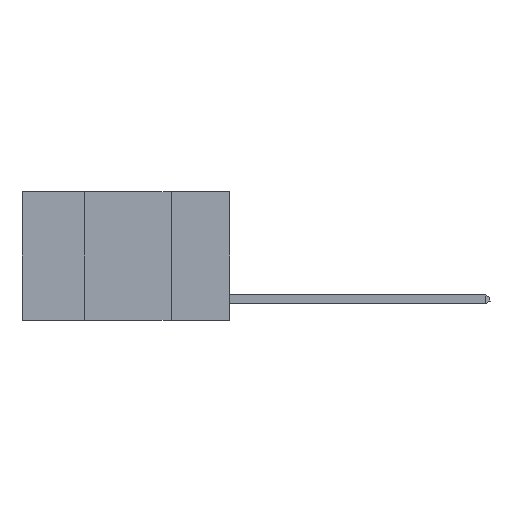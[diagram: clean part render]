
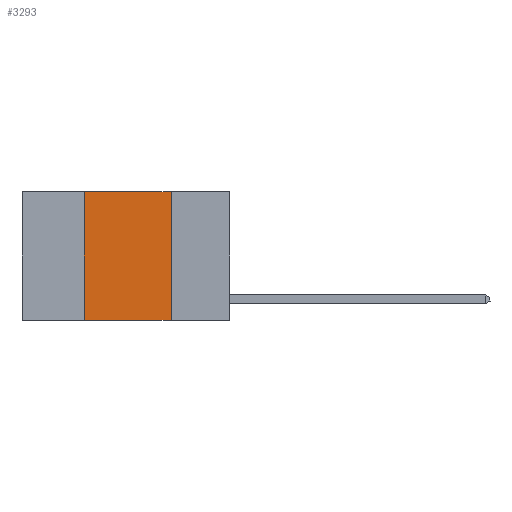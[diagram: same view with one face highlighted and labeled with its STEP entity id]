
A CAD part, left-side view. The second image highlights one B-rep face of the part: STEP entity #3293.
In plain terms, the highlighted planar face has unit normal (-1, 0, 0).
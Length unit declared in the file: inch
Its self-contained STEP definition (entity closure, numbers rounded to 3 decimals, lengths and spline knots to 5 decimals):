
#112 = AXIS2_PLACEMENT_3D ( 'NONE', #6970, #8048, #3590 ) ;
#480 = CARTESIAN_POINT ( 'NONE',  ( 0., 0.6, -0.37 ) ) ;
#869 = CARTESIAN_POINT ( 'NONE',  ( 0., 0.17, -0.37 ) ) ;
#885 = PLANE ( 'NONE',  #112 ) ;
#901 = ORIENTED_EDGE ( 'NONE', *, *, #1354, .F. ) ;
#1239 = LINE ( 'NONE', #4077, #8065 ) ;
#1354 = EDGE_CURVE ( 'NONE', #8734, #9245, #9266, .T. ) ;
#1361 = DIRECTION ( 'NONE',  ( 0., 0., -1. ) ) ;
#1508 = EDGE_CURVE ( 'NONE', #10641, #7084, #1239, .T. ) ;
#1574 = EDGE_LOOP ( 'NONE', ( #6700, #7855, #901, #9587 ) ) ;
#1585 = CARTESIAN_POINT ( 'NONE',  ( 0., 0.17, 0. ) ) ;
#2046 = VECTOR ( 'NONE', #9207, 39.37008 ) ;
#3048 = VECTOR ( 'NONE', #11203, 39.37008 ) ;
#3293 = ADVANCED_FACE ( 'NONE', ( #11440 ), #885, .F. ) ;
#3470 = VECTOR ( 'NONE', #4023, 39.37008 ) ;
#3590 = DIRECTION ( 'NONE',  ( 0., 0., -1. ) ) ;
#3980 = CARTESIAN_POINT ( 'NONE',  ( 0., 0.42, 0. ) ) ;
#4023 = DIRECTION ( 'NONE',  ( 0., -1., 0. ) ) ;
#4077 = CARTESIAN_POINT ( 'NONE',  ( 0., 0.17, 0. ) ) ;
#4091 = CARTESIAN_POINT ( 'NONE',  ( 0., 0.42, -0.37 ) ) ;
#4759 = CARTESIAN_POINT ( 'NONE',  ( 0., 0.6, 0. ) ) ;
#4962 = LINE ( 'NONE', #480, #3048 ) ;
#5036 = CARTESIAN_POINT ( 'NONE',  ( 0., 0.42, 0. ) ) ;
#6116 = EDGE_CURVE ( 'NONE', #8734, #7084, #4962, .T. ) ;
#6479 = LINE ( 'NONE', #4759, #3470 ) ;
#6700 = ORIENTED_EDGE ( 'NONE', *, *, #1508, .F. ) ;
#6970 = CARTESIAN_POINT ( 'NONE',  ( 0., 0.6, 0. ) ) ;
#7084 = VERTEX_POINT ( 'NONE', #869 ) ;
#7855 = ORIENTED_EDGE ( 'NONE', *, *, #10046, .F. ) ;
#8048 = DIRECTION ( 'NONE',  ( 1., 0., 0. ) ) ;
#8065 = VECTOR ( 'NONE', #1361, 39.37008 ) ;
#8734 = VERTEX_POINT ( 'NONE', #4091 ) ;
#9207 = DIRECTION ( 'NONE',  ( 0., 0., 1. ) ) ;
#9245 = VERTEX_POINT ( 'NONE', #5036 ) ;
#9266 = LINE ( 'NONE', #3980, #2046 ) ;
#9587 = ORIENTED_EDGE ( 'NONE', *, *, #6116, .T. ) ;
#10046 = EDGE_CURVE ( 'NONE', #9245, #10641, #6479, .T. ) ;
#10641 = VERTEX_POINT ( 'NONE', #1585 ) ;
#11203 = DIRECTION ( 'NONE',  ( 0., -1., 0. ) ) ;
#11440 = FACE_OUTER_BOUND ( 'NONE', #1574, .T. ) ;
